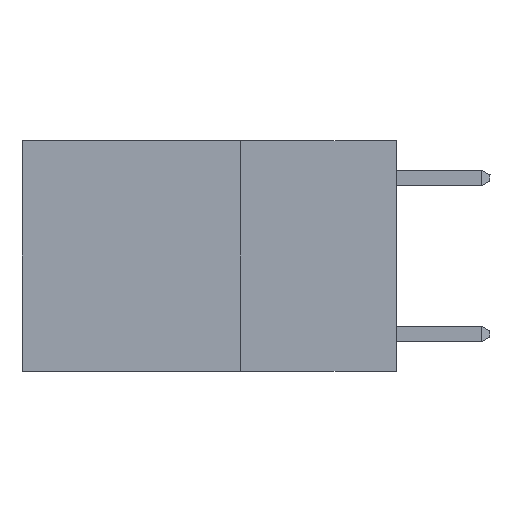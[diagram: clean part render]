
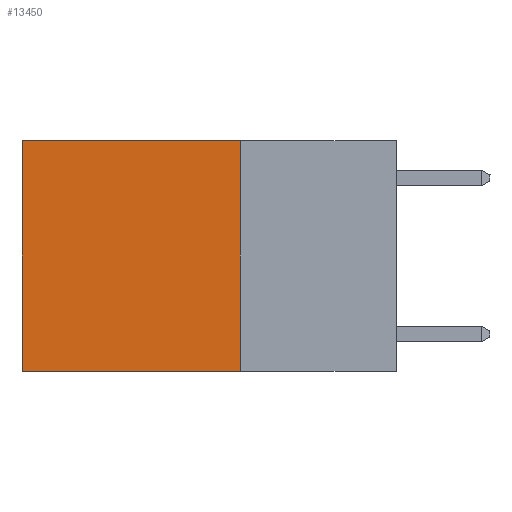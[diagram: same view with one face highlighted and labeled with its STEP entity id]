
A CAD part, left-side view. The second image highlights one B-rep face of the part: STEP entity #13450.
In plain terms, the highlighted planar face has unit normal (-1, 0, 0).
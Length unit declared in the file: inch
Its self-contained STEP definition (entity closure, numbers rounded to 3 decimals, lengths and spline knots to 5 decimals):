
#1216 = AXIS2_PLACEMENT_3D ( 'NONE', #3878, #13944, #7230 ) ;
#1335 = DIRECTION ( 'NONE',  ( 0., 0., -1. ) ) ;
#1902 = EDGE_CURVE ( 'NONE', #6658, #2715, #6967, .T. ) ;
#2216 = VECTOR ( 'NONE', #11811, 39.37008 ) ;
#2715 = VERTEX_POINT ( 'NONE', #6845 ) ;
#3275 = ORIENTED_EDGE ( 'NONE', *, *, #1902, .T. ) ;
#3878 = CARTESIAN_POINT ( 'NONE',  ( 0.2625, 0.25, 0. ) ) ;
#3982 = CARTESIAN_POINT ( 'NONE',  ( 0.2625, 0.25, -0.37 ) ) ;
#4369 = VECTOR ( 'NONE', #13000, 39.37008 ) ;
#4398 = EDGE_CURVE ( 'NONE', #11718, #6634, #8174, .T. ) ;
#5175 = CARTESIAN_POINT ( 'NONE',  ( 0.2625, 0.25, 0. ) ) ;
#5486 = VECTOR ( 'NONE', #1335, 39.37008 ) ;
#5555 = ORIENTED_EDGE ( 'NONE', *, *, #4398, .F. ) ;
#5678 = CARTESIAN_POINT ( 'NONE',  ( 0.2625, 0.6, -0.37 ) ) ;
#5839 = CARTESIAN_POINT ( 'NONE',  ( 0.2625, 0.6, 0. ) ) ;
#5885 = LINE ( 'NONE', #6884, #14446 ) ;
#6634 = VERTEX_POINT ( 'NONE', #5678 ) ;
#6658 = VERTEX_POINT ( 'NONE', #13537 ) ;
#6845 = CARTESIAN_POINT ( 'NONE',  ( 0.2625, 0.6, 0. ) ) ;
#6884 = CARTESIAN_POINT ( 'NONE',  ( 0.2625, 0.25, 0. ) ) ;
#6967 = LINE ( 'NONE', #5175, #4369 ) ;
#7230 = DIRECTION ( 'NONE',  ( 0., 0., -1. ) ) ;
#7282 = ORIENTED_EDGE ( 'NONE', *, *, #9608, .F. ) ;
#7405 = EDGE_CURVE ( 'NONE', #2715, #6634, #11766, .T. ) ;
#8174 = LINE ( 'NONE', #3982, #2216 ) ;
#9608 = EDGE_CURVE ( 'NONE', #6658, #11718, #5885, .T. ) ;
#9842 = CARTESIAN_POINT ( 'NONE',  ( 0.2625, 0.25, -0.37 ) ) ;
#10564 = FACE_OUTER_BOUND ( 'NONE', #12626, .T. ) ;
#11711 = PLANE ( 'NONE',  #1216 ) ;
#11718 = VERTEX_POINT ( 'NONE', #9842 ) ;
#11766 = LINE ( 'NONE', #5839, #5486 ) ;
#11811 = DIRECTION ( 'NONE',  ( 0., 1., 0. ) ) ;
#12506 = DIRECTION ( 'NONE',  ( 0., 0., -1. ) ) ;
#12626 = EDGE_LOOP ( 'NONE', ( #12984, #5555, #7282, #3275 ) ) ;
#12984 = ORIENTED_EDGE ( 'NONE', *, *, #7405, .T. ) ;
#13000 = DIRECTION ( 'NONE',  ( 0., 1., 0. ) ) ;
#13450 = ADVANCED_FACE ( 'NONE', ( #10564 ), #11711, .F. ) ;
#13537 = CARTESIAN_POINT ( 'NONE',  ( 0.2625, 0.25, 0. ) ) ;
#13944 = DIRECTION ( 'NONE',  ( 1., 0., 0. ) ) ;
#14446 = VECTOR ( 'NONE', #12506, 39.37008 ) ;
